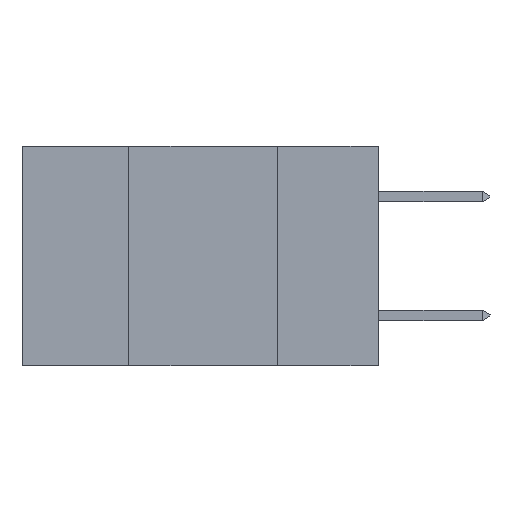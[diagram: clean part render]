
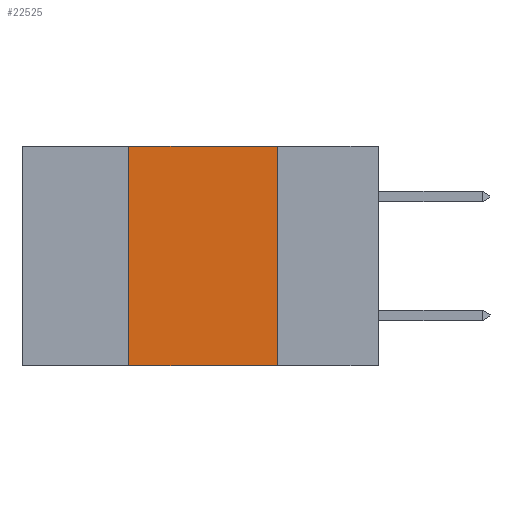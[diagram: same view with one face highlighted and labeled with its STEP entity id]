
A CAD part, left-side view. The second image highlights one B-rep face of the part: STEP entity #22525.
In plain terms, the highlighted planar face has unit normal (-1, 0, 0).
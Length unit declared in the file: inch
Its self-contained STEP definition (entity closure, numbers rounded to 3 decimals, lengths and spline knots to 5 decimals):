
#233 = VERTEX_POINT ( 'NONE', #12755 ) ;
#1172 = CARTESIAN_POINT ( 'NONE',  ( 0., 0.17, -0.37 ) ) ;
#1574 = PLANE ( 'NONE',  #18091 ) ;
#2666 = LINE ( 'NONE', #1172, #17749 ) ;
#2761 = FACE_OUTER_BOUND ( 'NONE', #9821, .T. ) ;
#3535 = VERTEX_POINT ( 'NONE', #9160 ) ;
#3701 = CARTESIAN_POINT ( 'NONE',  ( 0., 0.42, -0.37 ) ) ;
#4106 = VERTEX_POINT ( 'NONE', #15011 ) ;
#5041 = DIRECTION ( 'NONE',  ( 0., -1., 0. ) ) ;
#5550 = CARTESIAN_POINT ( 'NONE',  ( 0., 0.6, 0. ) ) ;
#6684 = EDGE_CURVE ( 'NONE', #7572, #3535, #2666, .T. ) ;
#7116 = CARTESIAN_POINT ( 'NONE',  ( 0., 0.6, -0.37 ) ) ;
#7509 = DIRECTION ( 'NONE',  ( 0., 0., -1. ) ) ;
#7572 = VERTEX_POINT ( 'NONE', #19290 ) ;
#8747 = ORIENTED_EDGE ( 'NONE', *, *, #9327, .F. ) ;
#8758 = VECTOR ( 'NONE', #5041, 39.37008 ) ;
#9160 = CARTESIAN_POINT ( 'NONE',  ( 0., 0.17, -0.37 ) ) ;
#9327 = EDGE_CURVE ( 'NONE', #233, #7572, #19227, .T. ) ;
#9821 = EDGE_LOOP ( 'NONE', ( #24115, #8747, #19217, #21065 ) ) ;
#12249 = VECTOR ( 'NONE', #19446, 39.37008 ) ;
#12755 = CARTESIAN_POINT ( 'NONE',  ( 0., 0.42, 0. ) ) ;
#12877 = CARTESIAN_POINT ( 'NONE',  ( 0., 0.6, 0. ) ) ;
#13949 = VECTOR ( 'NONE', #22823, 39.37008 ) ;
#14976 = DIRECTION ( 'NONE',  ( 0., 0., -1. ) ) ;
#15011 = CARTESIAN_POINT ( 'NONE',  ( 0., 0.42, -0.37 ) ) ;
#15952 = EDGE_CURVE ( 'NONE', #4106, #233, #22666, .T. ) ;
#17749 = VECTOR ( 'NONE', #14976, 39.37008 ) ;
#18091 = AXIS2_PLACEMENT_3D ( 'NONE', #5550, #19289, #7509 ) ;
#19217 = ORIENTED_EDGE ( 'NONE', *, *, #15952, .F. ) ;
#19227 = LINE ( 'NONE', #12877, #8758 ) ;
#19289 = DIRECTION ( 'NONE',  ( 1., 0., 0. ) ) ;
#19290 = CARTESIAN_POINT ( 'NONE',  ( 0., 0.17, 0. ) ) ;
#19446 = DIRECTION ( 'NONE',  ( 0., 0., 1. ) ) ;
#21065 = ORIENTED_EDGE ( 'NONE', *, *, #21181, .T. ) ;
#21181 = EDGE_CURVE ( 'NONE', #4106, #3535, #24303, .T. ) ;
#22525 = ADVANCED_FACE ( 'NONE', ( #2761 ), #1574, .F. ) ;
#22666 = LINE ( 'NONE', #3701, #12249 ) ;
#22823 = DIRECTION ( 'NONE',  ( 0., -1., 0. ) ) ;
#24115 = ORIENTED_EDGE ( 'NONE', *, *, #6684, .F. ) ;
#24303 = LINE ( 'NONE', #7116, #13949 ) ;
